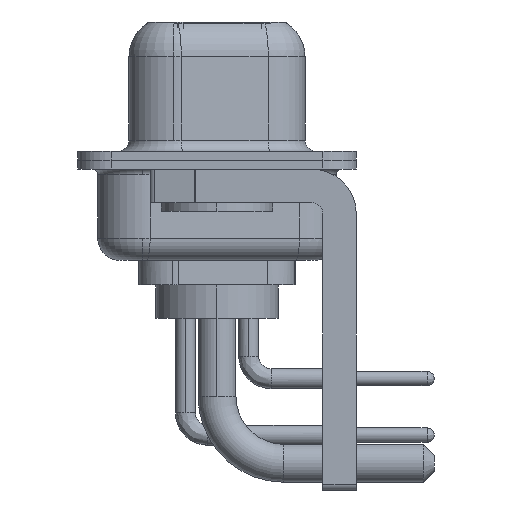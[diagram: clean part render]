
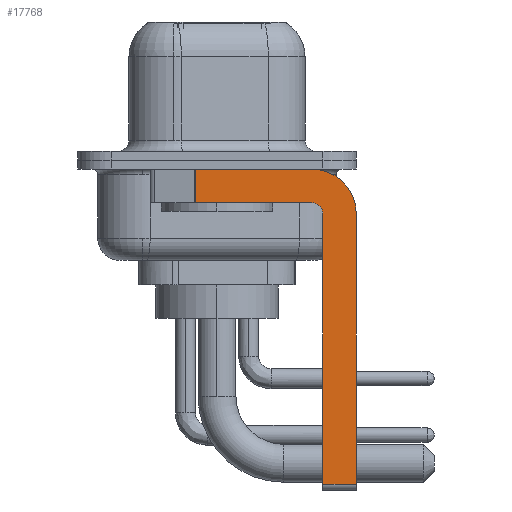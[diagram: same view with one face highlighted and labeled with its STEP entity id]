
A CAD part, left-side view. The second image highlights one B-rep face of the part: STEP entity #17768.
In plain terms, the highlighted planar face has unit normal (-1, 0, 0).
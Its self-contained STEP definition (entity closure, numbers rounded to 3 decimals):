
#315 = CARTESIAN_POINT ( 'NONE',  ( -2.9, -4.75, -14.55 ) ) ;
#523 = CARTESIAN_POINT ( 'NONE',  ( -2.9, 0.978, -1.9 ) ) ;
#1009 = CARTESIAN_POINT ( 'NONE',  ( -2.9, -4.25, -1.9 ) ) ;
#1327 = CARTESIAN_POINT ( 'NONE',  ( -2.9, -6.25, -2.4 ) ) ;
#1912 = LINE ( 'NONE', #11168, #18519 ) ;
#2133 = DIRECTION ( 'NONE',  ( 0., 1., 0. ) ) ;
#2576 = VECTOR ( 'NONE', #12825, 1000. ) ;
#3097 = DIRECTION ( 'NONE',  ( 0., -1., 0. ) ) ;
#3147 = CIRCLE ( 'NONE', #15025, 0.5 ) ;
#3676 = VERTEX_POINT ( 'NONE', #20600 ) ;
#3719 = LINE ( 'NONE', #10200, #4315 ) ;
#3887 = VERTEX_POINT ( 'NONE', #20549 ) ;
#4002 = ORIENTED_EDGE ( 'NONE', *, *, #5074, .F. ) ;
#4315 = VECTOR ( 'NONE', #15104, 1000. ) ;
#4590 = CARTESIAN_POINT ( 'NONE',  ( -2.9, -4.25, -2.4 ) ) ;
#4699 = VERTEX_POINT ( 'NONE', #8902 ) ;
#4857 = LINE ( 'NONE', #6547, #2576 ) ;
#5074 = EDGE_CURVE ( 'NONE', #10350, #4699, #4857, .T. ) ;
#5326 = EDGE_CURVE ( 'NONE', #3676, #14418, #10692, .T. ) ;
#5452 = ORIENTED_EDGE ( 'NONE', *, *, #12274, .F. ) ;
#5934 = DIRECTION ( 'NONE',  ( 0., 0., -1. ) ) ;
#6057 = CARTESIAN_POINT ( 'NONE',  ( -2.9, -4.25, -2.4 ) ) ;
#6179 = ORIENTED_EDGE ( 'NONE', *, *, #5326, .F. ) ;
#6206 = ORIENTED_EDGE ( 'NONE', *, *, #13351, .F. ) ;
#6547 = CARTESIAN_POINT ( 'NONE',  ( -2.9, -4.75, -14.8 ) ) ;
#6818 = LINE ( 'NONE', #10532, #20842 ) ;
#6884 = CIRCLE ( 'NONE', #14740, 2. ) ;
#7054 = EDGE_LOOP ( 'NONE', ( #13571, #18472, #6206, #19100, #4002, #13365, #6179, #5452 ) ) ;
#7566 = EDGE_CURVE ( 'NONE', #13870, #3887, #3719, .T. ) ;
#7851 = DIRECTION ( 'NONE',  ( 0., 0., -1. ) ) ;
#8594 = DIRECTION ( 'NONE',  ( 0., 0., -1. ) ) ;
#8900 = DIRECTION ( 'NONE',  ( 1., 0., 0. ) ) ;
#8902 = CARTESIAN_POINT ( 'NONE',  ( -2.9, -4.75, -2.4 ) ) ;
#8937 = CARTESIAN_POINT ( 'NONE',  ( -2.9, 0.978, -1.9 ) ) ;
#10200 = CARTESIAN_POINT ( 'NONE',  ( -2.9, 3., -0.4 ) ) ;
#10284 = EDGE_CURVE ( 'NONE', #4699, #18685, #3147, .T. ) ;
#10350 = VERTEX_POINT ( 'NONE', #315 ) ;
#10421 = EDGE_CURVE ( 'NONE', #13870, #19927, #18478, .T. ) ;
#10532 = CARTESIAN_POINT ( 'NONE',  ( -2.9, -4.25, -1.9 ) ) ;
#10692 = LINE ( 'NONE', #1327, #12074 ) ;
#11168 = CARTESIAN_POINT ( 'NONE',  ( -2.9, -4.25, -14.55 ) ) ;
#11780 = CARTESIAN_POINT ( 'NONE',  ( -2.9, 0.978, -0.4 ) ) ;
#12074 = VECTOR ( 'NONE', #13983, 1000. ) ;
#12274 = EDGE_CURVE ( 'NONE', #3887, #3676, #6884, .T. ) ;
#12825 = DIRECTION ( 'NONE',  ( 0., 0., 1. ) ) ;
#13351 = EDGE_CURVE ( 'NONE', #18685, #19927, #6818, .T. ) ;
#13365 = ORIENTED_EDGE ( 'NONE', *, *, #15125, .T. ) ;
#13571 = ORIENTED_EDGE ( 'NONE', *, *, #7566, .F. ) ;
#13870 = VERTEX_POINT ( 'NONE', #11780 ) ;
#13983 = DIRECTION ( 'NONE',  ( 0., 0., -1. ) ) ;
#14418 = VERTEX_POINT ( 'NONE', #15489 ) ;
#14576 = DIRECTION ( 'NONE',  ( -1., 0., 0. ) ) ;
#14740 = AXIS2_PLACEMENT_3D ( 'NONE', #20274, #8900, #5934 ) ;
#14852 = AXIS2_PLACEMENT_3D ( 'NONE', #6057, #19209, #7851 ) ;
#15025 = AXIS2_PLACEMENT_3D ( 'NONE', #4590, #14576, #19538 ) ;
#15104 = DIRECTION ( 'NONE',  ( 0., -1., 0. ) ) ;
#15125 = EDGE_CURVE ( 'NONE', #10350, #14418, #1912, .T. ) ;
#15443 = PLANE ( 'NONE',  #14852 ) ;
#15489 = CARTESIAN_POINT ( 'NONE',  ( -2.9, -6.25, -14.55 ) ) ;
#16366 = VECTOR ( 'NONE', #8594, 1000. ) ;
#17768 = ADVANCED_FACE ( 'NONE', ( #19010 ), #15443, .F. ) ;
#18472 = ORIENTED_EDGE ( 'NONE', *, *, #10421, .T. ) ;
#18478 = LINE ( 'NONE', #523, #16366 ) ;
#18519 = VECTOR ( 'NONE', #3097, 1000. ) ;
#18685 = VERTEX_POINT ( 'NONE', #1009 ) ;
#19010 = FACE_OUTER_BOUND ( 'NONE', #7054, .T. ) ;
#19100 = ORIENTED_EDGE ( 'NONE', *, *, #10284, .F. ) ;
#19209 = DIRECTION ( 'NONE',  ( 1., 0., 0. ) ) ;
#19538 = DIRECTION ( 'NONE',  ( 0., 0., 1. ) ) ;
#19927 = VERTEX_POINT ( 'NONE', #8937 ) ;
#20274 = CARTESIAN_POINT ( 'NONE',  ( -2.9, -4.25, -2.4 ) ) ;
#20549 = CARTESIAN_POINT ( 'NONE',  ( -2.9, -4.25, -0.4 ) ) ;
#20600 = CARTESIAN_POINT ( 'NONE',  ( -2.9, -6.25, -2.4 ) ) ;
#20842 = VECTOR ( 'NONE', #2133, 1000. ) ;
